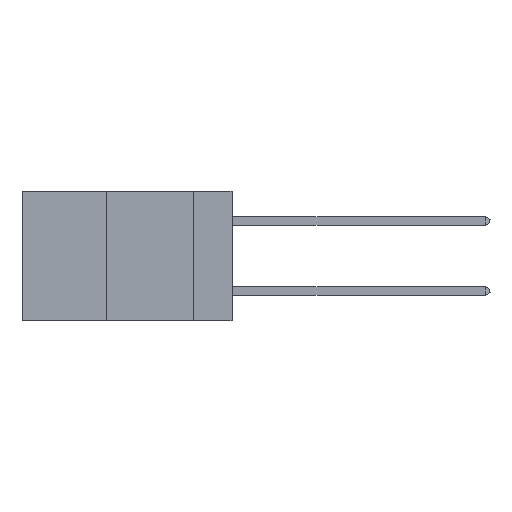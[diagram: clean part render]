
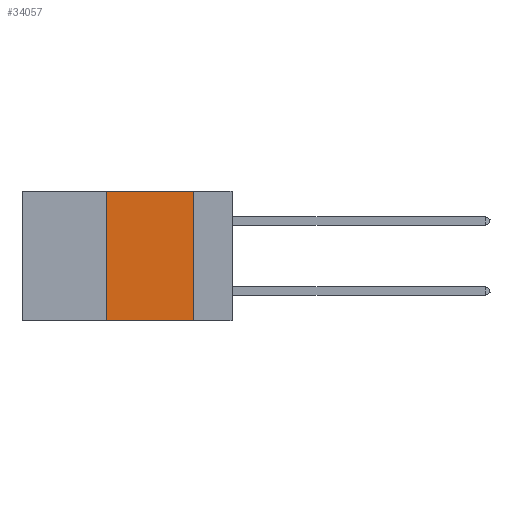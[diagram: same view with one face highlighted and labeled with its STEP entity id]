
A CAD part, left-side view. The second image highlights one B-rep face of the part: STEP entity #34057.
In plain terms, the highlighted planar face has unit normal (-1, 0, 0).
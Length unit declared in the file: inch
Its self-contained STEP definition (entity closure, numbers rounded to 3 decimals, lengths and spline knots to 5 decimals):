
#3265 = EDGE_LOOP ( 'NONE', ( #16492, #7793, #29810, #11298 ) ) ;
#3782 = DIRECTION ( 'NONE',  ( 1., 0., 0. ) ) ;
#4795 = CARTESIAN_POINT ( 'NONE',  ( 0., 0.36, 0. ) ) ;
#5579 = LINE ( 'NONE', #20831, #33976 ) ;
#7114 = CARTESIAN_POINT ( 'NONE',  ( 0., 0.36, -0.37 ) ) ;
#7793 = ORIENTED_EDGE ( 'NONE', *, *, #30665, .F. ) ;
#11207 = CARTESIAN_POINT ( 'NONE',  ( 0., 0.6, 0. ) ) ;
#11298 = ORIENTED_EDGE ( 'NONE', *, *, #15040, .T. ) ;
#14655 = LINE ( 'NONE', #25364, #32018 ) ;
#14942 = CARTESIAN_POINT ( 'NONE',  ( 0., 0.11, 0. ) ) ;
#15040 = EDGE_CURVE ( 'NONE', #23547, #29821, #5579, .T. ) ;
#16492 = ORIENTED_EDGE ( 'NONE', *, *, #42145, .F. ) ;
#17181 = AXIS2_PLACEMENT_3D ( 'NONE', #11207, #3782, #29794 ) ;
#18958 = VERTEX_POINT ( 'NONE', #31063 ) ;
#20077 = VECTOR ( 'NONE', #27061, 39.37008 ) ;
#20831 = CARTESIAN_POINT ( 'NONE',  ( 0., 0.6, -0.37 ) ) ;
#21805 = DIRECTION ( 'NONE',  ( 0., -1., 0. ) ) ;
#23547 = VERTEX_POINT ( 'NONE', #7114 ) ;
#24536 = DIRECTION ( 'NONE',  ( 0., -1., 0. ) ) ;
#24561 = LINE ( 'NONE', #14942, #35504 ) ;
#25364 = CARTESIAN_POINT ( 'NONE',  ( 0., 0.6, 0. ) ) ;
#27061 = DIRECTION ( 'NONE',  ( 0., 0., 1. ) ) ;
#29794 = DIRECTION ( 'NONE',  ( 0., 0., -1. ) ) ;
#29810 = ORIENTED_EDGE ( 'NONE', *, *, #40942, .F. ) ;
#29821 = VERTEX_POINT ( 'NONE', #47489 ) ;
#30655 = VERTEX_POINT ( 'NONE', #36302 ) ;
#30665 = EDGE_CURVE ( 'NONE', #30655, #18958, #14655, .T. ) ;
#31063 = CARTESIAN_POINT ( 'NONE',  ( 0., 0.11, 0. ) ) ;
#32018 = VECTOR ( 'NONE', #21805, 39.37008 ) ;
#33976 = VECTOR ( 'NONE', #24536, 39.37008 ) ;
#34057 = ADVANCED_FACE ( 'NONE', ( #34592 ), #44359, .F. ) ;
#34592 = FACE_OUTER_BOUND ( 'NONE', #3265, .T. ) ;
#35504 = VECTOR ( 'NONE', #40751, 39.37008 ) ;
#36302 = CARTESIAN_POINT ( 'NONE',  ( 0., 0.36, 0. ) ) ;
#39619 = LINE ( 'NONE', #4795, #20077 ) ;
#40751 = DIRECTION ( 'NONE',  ( 0., 0., -1. ) ) ;
#40942 = EDGE_CURVE ( 'NONE', #23547, #30655, #39619, .T. ) ;
#42145 = EDGE_CURVE ( 'NONE', #18958, #29821, #24561, .T. ) ;
#44359 = PLANE ( 'NONE',  #17181 ) ;
#47489 = CARTESIAN_POINT ( 'NONE',  ( 0., 0.11, -0.37 ) ) ;
